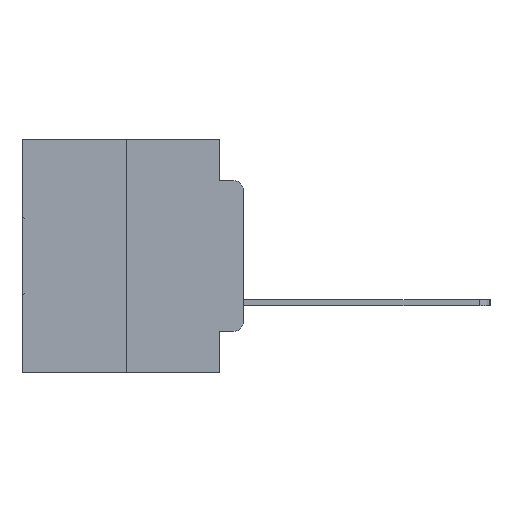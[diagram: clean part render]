
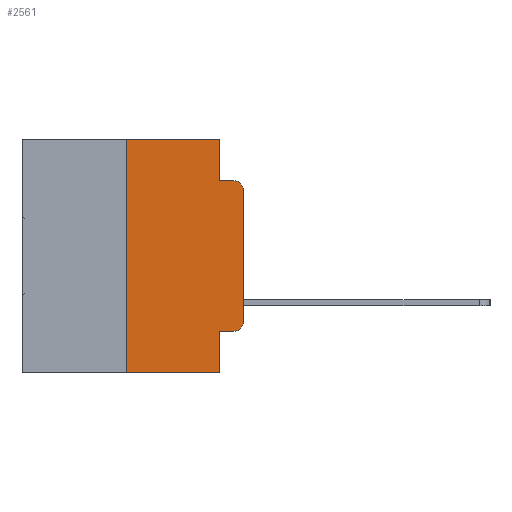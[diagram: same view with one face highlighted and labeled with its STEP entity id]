
A CAD part, left-side view. The second image highlights one B-rep face of the part: STEP entity #2561.
In plain terms, the highlighted planar face has unit normal (-1, 0, 0).
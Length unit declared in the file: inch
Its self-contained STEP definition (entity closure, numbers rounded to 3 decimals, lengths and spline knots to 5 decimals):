
#148 = VERTEX_POINT ( 'NONE', #10790 ) ;
#1044 = EDGE_CURVE ( 'NONE', #148, #26423, #22393, .T. ) ;
#1897 = EDGE_CURVE ( 'NONE', #8199, #4760, #12582, .T. ) ;
#2561 = ADVANCED_FACE ( 'NONE', ( #24164 ), #12945, .F. ) ;
#2900 = DIRECTION ( 'NONE',  ( 0., 0., 1. ) ) ;
#2968 = CARTESIAN_POINT ( 'NONE',  ( 0., 0.02, -0.0885 ) ) ;
#3811 = VECTOR ( 'NONE', #14801, 39.37008 ) ;
#3974 = CARTESIAN_POINT ( 'NONE',  ( 0., 0.051, 0. ) ) ;
#3994 = AXIS2_PLACEMENT_3D ( 'NONE', #25110, #10802, #27430 ) ;
#4025 = DIRECTION ( 'NONE',  ( 0., -1., 0. ) ) ;
#4537 = VECTOR ( 'NONE', #2900, 39.37008 ) ;
#4672 = ORIENTED_EDGE ( 'NONE', *, *, #12992, .F. ) ;
#4674 = VECTOR ( 'NONE', #12638, 39.37008 ) ;
#4760 = VERTEX_POINT ( 'NONE', #15585 ) ;
#5359 = CARTESIAN_POINT ( 'NONE',  ( 0., 0.473, 0. ) ) ;
#6225 = VERTEX_POINT ( 'NONE', #16211 ) ;
#6791 = VECTOR ( 'NONE', #4025, 39.37008 ) ;
#6968 = ORIENTED_EDGE ( 'NONE', *, *, #9088, .T. ) ;
#7157 = AXIS2_PLACEMENT_3D ( 'NONE', #13661, #30128, #16068 ) ;
#7265 = LINE ( 'NONE', #11598, #30343 ) ;
#7631 = CARTESIAN_POINT ( 'NONE',  ( 0., 0.051, -0.5 ) ) ;
#8199 = VERTEX_POINT ( 'NONE', #25744 ) ;
#9008 = CARTESIAN_POINT ( 'NONE',  ( 0., 0.25, -0.5 ) ) ;
#9088 = EDGE_CURVE ( 'NONE', #26423, #8199, #25368, .T. ) ;
#9420 = VERTEX_POINT ( 'NONE', #7631 ) ;
#9579 = VECTOR ( 'NONE', #25930, 39.37008 ) ;
#9812 = VERTEX_POINT ( 'NONE', #9008 ) ;
#9853 = EDGE_CURVE ( 'NONE', #9812, #9420, #12809, .T. ) ;
#10014 = CARTESIAN_POINT ( 'NONE',  ( 0., 0.051, -0.0885 ) ) ;
#10790 = CARTESIAN_POINT ( 'NONE',  ( 0., 0.051, -0.4115 ) ) ;
#10802 = DIRECTION ( 'NONE',  ( -1., 0., 0. ) ) ;
#11380 = DIRECTION ( 'NONE',  ( 0., 0., -1. ) ) ;
#11598 = CARTESIAN_POINT ( 'NONE',  ( 0., 0.25, 0. ) ) ;
#11714 = DIRECTION ( 'NONE',  ( 0., -1., 0. ) ) ;
#11912 = EDGE_CURVE ( 'NONE', #6225, #28685, #23973, .T. ) ;
#12380 = CARTESIAN_POINT ( 'NONE',  ( 0., 0.051, 0. ) ) ;
#12465 = EDGE_LOOP ( 'NONE', ( #14589, #27209, #16098, #22474, #16853, #4672, #30056, #24697, #30768, #6968 ) ) ;
#12582 = LINE ( 'NONE', #24593, #4537 ) ;
#12638 = DIRECTION ( 'NONE',  ( 0., -1., 0. ) ) ;
#12809 = LINE ( 'NONE', #25992, #30141 ) ;
#12945 = PLANE ( 'NONE',  #17211 ) ;
#12992 = EDGE_CURVE ( 'NONE', #9812, #6225, #7265, .T. ) ;
#13110 = CIRCLE ( 'NONE', #3994, 0.02 ) ;
#13661 = CARTESIAN_POINT ( 'NONE',  ( 0., 0.02, -0.3915 ) ) ;
#14589 = ORIENTED_EDGE ( 'NONE', *, *, #1897, .T. ) ;
#14801 = DIRECTION ( 'NONE',  ( 0., 0., -1. ) ) ;
#15351 = DIRECTION ( 'NONE',  ( 0., 0., -1. ) ) ;
#15585 = CARTESIAN_POINT ( 'NONE',  ( 0., 0., -0.1085 ) ) ;
#16068 = DIRECTION ( 'NONE',  ( 0., 0., -1. ) ) ;
#16098 = ORIENTED_EDGE ( 'NONE', *, *, #29792, .F. ) ;
#16211 = CARTESIAN_POINT ( 'NONE',  ( 0., 0.25, 0. ) ) ;
#16512 = LINE ( 'NONE', #3974, #17244 ) ;
#16853 = ORIENTED_EDGE ( 'NONE', *, *, #11912, .F. ) ;
#17211 = AXIS2_PLACEMENT_3D ( 'NONE', #27064, #29454, #15351 ) ;
#17244 = VECTOR ( 'NONE', #11380, 39.37008 ) ;
#18253 = LINE ( 'NONE', #12380, #3811 ) ;
#18284 = CARTESIAN_POINT ( 'NONE',  ( 0., 0.02, -0.4115 ) ) ;
#18855 = DIRECTION ( 'NONE',  ( 0., 0., 1. ) ) ;
#20417 = EDGE_CURVE ( 'NONE', #28685, #30070, #18253, .T. ) ;
#21176 = LINE ( 'NONE', #25607, #6791 ) ;
#22393 = LINE ( 'NONE', #28248, #9579 ) ;
#22474 = ORIENTED_EDGE ( 'NONE', *, *, #20417, .F. ) ;
#22631 = EDGE_CURVE ( 'NONE', #148, #9420, #16512, .T. ) ;
#23640 = EDGE_CURVE ( 'NONE', #4760, #28132, #13110, .T. ) ;
#23973 = LINE ( 'NONE', #5359, #4674 ) ;
#24164 = FACE_OUTER_BOUND ( 'NONE', #12465, .T. ) ;
#24593 = CARTESIAN_POINT ( 'NONE',  ( 0., 0., 0. ) ) ;
#24697 = ORIENTED_EDGE ( 'NONE', *, *, #22631, .F. ) ;
#25018 = CARTESIAN_POINT ( 'NONE',  ( 0., 0.051, 0. ) ) ;
#25110 = CARTESIAN_POINT ( 'NONE',  ( 0., 0.02, -0.1085 ) ) ;
#25368 = CIRCLE ( 'NONE', #7157, 0.02 ) ;
#25607 = CARTESIAN_POINT ( 'NONE',  ( 0., 0.051, -0.0885 ) ) ;
#25744 = CARTESIAN_POINT ( 'NONE',  ( 0., 0., -0.3915 ) ) ;
#25930 = DIRECTION ( 'NONE',  ( 0., -1., 0. ) ) ;
#25992 = CARTESIAN_POINT ( 'NONE',  ( 0., 0.473, -0.5 ) ) ;
#26423 = VERTEX_POINT ( 'NONE', #18284 ) ;
#27064 = CARTESIAN_POINT ( 'NONE',  ( 0., 0.473, 0. ) ) ;
#27209 = ORIENTED_EDGE ( 'NONE', *, *, #23640, .T. ) ;
#27430 = DIRECTION ( 'NONE',  ( 0., 0., -1. ) ) ;
#28132 = VERTEX_POINT ( 'NONE', #2968 ) ;
#28248 = CARTESIAN_POINT ( 'NONE',  ( 0., 0.051, -0.4115 ) ) ;
#28685 = VERTEX_POINT ( 'NONE', #25018 ) ;
#29454 = DIRECTION ( 'NONE',  ( 1., 0., 0. ) ) ;
#29792 = EDGE_CURVE ( 'NONE', #30070, #28132, #21176, .T. ) ;
#30056 = ORIENTED_EDGE ( 'NONE', *, *, #9853, .T. ) ;
#30070 = VERTEX_POINT ( 'NONE', #10014 ) ;
#30128 = DIRECTION ( 'NONE',  ( -1., 0., 0. ) ) ;
#30141 = VECTOR ( 'NONE', #11714, 39.37008 ) ;
#30343 = VECTOR ( 'NONE', #18855, 39.37008 ) ;
#30768 = ORIENTED_EDGE ( 'NONE', *, *, #1044, .T. ) ;
